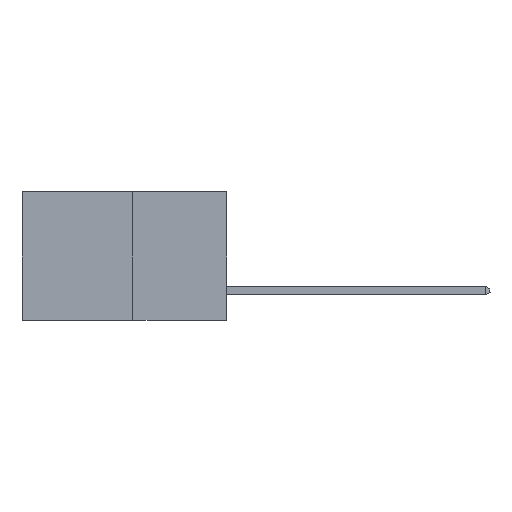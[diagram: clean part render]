
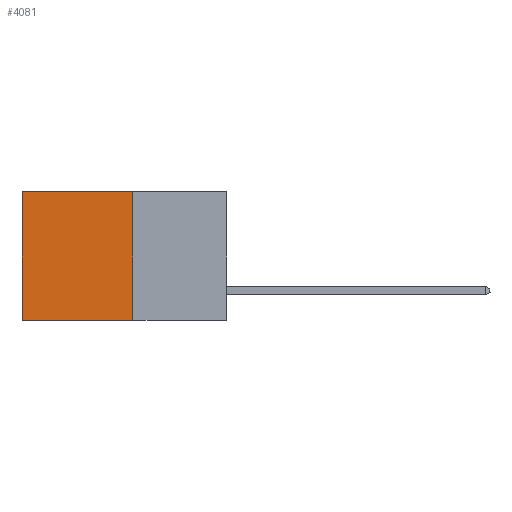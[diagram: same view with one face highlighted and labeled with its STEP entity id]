
A CAD part, left-side view. The second image highlights one B-rep face of the part: STEP entity #4081.
In plain terms, the highlighted planar face has unit normal (-1, 0, 0).
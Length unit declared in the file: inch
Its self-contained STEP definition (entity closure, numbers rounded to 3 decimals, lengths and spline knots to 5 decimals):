
#860 = CARTESIAN_POINT ( 'NONE',  ( 0.277, 0.59, 0. ) ) ;
#934 = ORIENTED_EDGE ( 'NONE', *, *, #4091, .F. ) ;
#1860 = VERTEX_POINT ( 'NONE', #12930 ) ;
#2710 = DIRECTION ( 'NONE',  ( 0., 0., -1. ) ) ;
#3197 = ORIENTED_EDGE ( 'NONE', *, *, #7923, .T. ) ;
#3709 = DIRECTION ( 'NONE',  ( 0., 0., -1. ) ) ;
#4081 = ADVANCED_FACE ( 'NONE', ( #14606 ), #7707, .F. ) ;
#4091 = EDGE_CURVE ( 'NONE', #1860, #11855, #8706, .T. ) ;
#4233 = VECTOR ( 'NONE', #3709, 39.37008 ) ;
#4883 = CARTESIAN_POINT ( 'NONE',  ( 0.277, 0.59, -0.37 ) ) ;
#7514 = CARTESIAN_POINT ( 'NONE',  ( 0.277, 0.27, -0.37 ) ) ;
#7670 = DIRECTION ( 'NONE',  ( 0., 0., -1. ) ) ;
#7673 = DIRECTION ( 'NONE',  ( 1., 0., 0. ) ) ;
#7707 = PLANE ( 'NONE',  #14916 ) ;
#7760 = DIRECTION ( 'NONE',  ( 0., 1., 0. ) ) ;
#7923 = EDGE_CURVE ( 'NONE', #13528, #9029, #10482, .T. ) ;
#7954 = CARTESIAN_POINT ( 'NONE',  ( 0.277, 0.27, -0.37 ) ) ;
#8082 = EDGE_LOOP ( 'NONE', ( #13734, #934, #12735, #3197 ) ) ;
#8706 = LINE ( 'NONE', #7514, #9075 ) ;
#9029 = VERTEX_POINT ( 'NONE', #860 ) ;
#9075 = VECTOR ( 'NONE', #7760, 39.37008 ) ;
#10482 = LINE ( 'NONE', #11580, #13456 ) ;
#10772 = LINE ( 'NONE', #4883, #4233 ) ;
#11055 = VECTOR ( 'NONE', #2710, 39.37008 ) ;
#11580 = CARTESIAN_POINT ( 'NONE',  ( 0.277, 0.27, 0. ) ) ;
#11754 = EDGE_CURVE ( 'NONE', #9029, #11855, #10772, .T. ) ;
#11855 = VERTEX_POINT ( 'NONE', #11945 ) ;
#11945 = CARTESIAN_POINT ( 'NONE',  ( 0.277, 0.59, -0.37 ) ) ;
#12689 = DIRECTION ( 'NONE',  ( 0., 1., 0. ) ) ;
#12735 = ORIENTED_EDGE ( 'NONE', *, *, #14851, .F. ) ;
#12930 = CARTESIAN_POINT ( 'NONE',  ( 0.277, 0.27, -0.37 ) ) ;
#13456 = VECTOR ( 'NONE', #12689, 39.37008 ) ;
#13528 = VERTEX_POINT ( 'NONE', #13949 ) ;
#13734 = ORIENTED_EDGE ( 'NONE', *, *, #11754, .T. ) ;
#13949 = CARTESIAN_POINT ( 'NONE',  ( 0.277, 0.27, 0. ) ) ;
#13985 = LINE ( 'NONE', #14182, #11055 ) ;
#14182 = CARTESIAN_POINT ( 'NONE',  ( 0.277, 0.27, -0.37 ) ) ;
#14606 = FACE_OUTER_BOUND ( 'NONE', #8082, .T. ) ;
#14851 = EDGE_CURVE ( 'NONE', #13528, #1860, #13985, .T. ) ;
#14916 = AXIS2_PLACEMENT_3D ( 'NONE', #7954, #7673, #7670 ) ;
